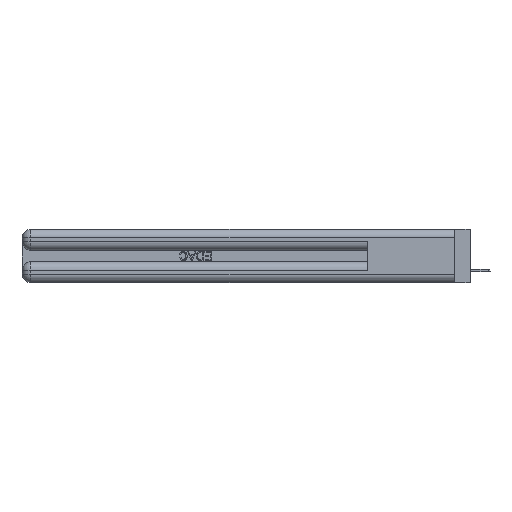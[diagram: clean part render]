
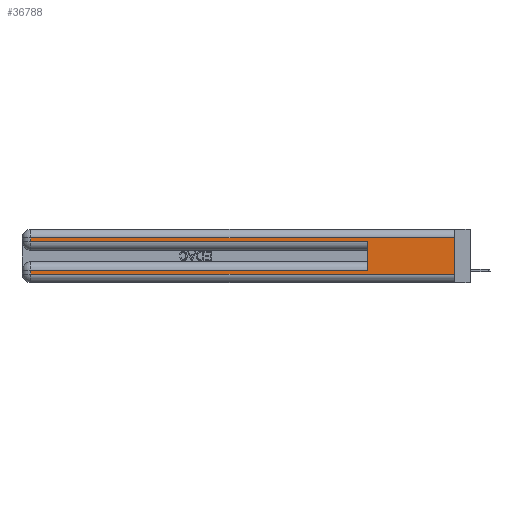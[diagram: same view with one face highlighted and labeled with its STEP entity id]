
A CAD part, left-side view. The second image highlights one B-rep face of the part: STEP entity #36788.
In plain terms, the highlighted planar face has unit normal (-1, 0, 0).
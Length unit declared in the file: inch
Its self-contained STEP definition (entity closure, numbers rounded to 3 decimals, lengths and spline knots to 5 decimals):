
#344 = CARTESIAN_POINT ( 'NONE',  ( 0., 0., 0.31 ) ) ;
#729 = CARTESIAN_POINT ( 'NONE',  ( 0., 0., 0.37 ) ) ;
#1096 = DIRECTION ( 'NONE',  ( 0., -1., 0. ) ) ;
#1603 = ORIENTED_EDGE ( 'NONE', *, *, #17889, .T. ) ;
#2224 = VERTEX_POINT ( 'NONE', #2836 ) ;
#2836 = CARTESIAN_POINT ( 'NONE',  ( 0., 0., 0.31 ) ) ;
#4087 = CARTESIAN_POINT ( 'NONE',  ( 0., 2.94, 0.06 ) ) ;
#6194 = CARTESIAN_POINT ( 'NONE',  ( 0., 2.94, 0.37 ) ) ;
#6710 = EDGE_CURVE ( 'NONE', #2224, #46949, #38378, .T. ) ;
#6787 = LINE ( 'NONE', #35916, #14885 ) ;
#9038 = EDGE_LOOP ( 'NONE', ( #23995, #1603, #45096, #53642, #51712, #34278, #30281, #24476 ) ) ;
#10480 = DIRECTION ( 'NONE',  ( 0., 1., 0. ) ) ;
#11946 = DIRECTION ( 'NONE',  ( 0., 1., 0. ) ) ;
#12211 = LINE ( 'NONE', #344, #42393 ) ;
#12593 = CARTESIAN_POINT ( 'NONE',  ( 0., 0., 0.37 ) ) ;
#14110 = EDGE_CURVE ( 'NONE', #15818, #34811, #22847, .T. ) ;
#14450 = DIRECTION ( 'NONE',  ( 0., 0., -1. ) ) ;
#14874 = EDGE_CURVE ( 'NONE', #15818, #25342, #43784, .T. ) ;
#14885 = VECTOR ( 'NONE', #52134, 39.37008 ) ;
#15342 = CARTESIAN_POINT ( 'NONE',  ( 0., 0.6, 0.085 ) ) ;
#15780 = CARTESIAN_POINT ( 'NONE',  ( 0., 0., 0.06 ) ) ;
#15818 = VERTEX_POINT ( 'NONE', #15342 ) ;
#16564 = EDGE_CURVE ( 'NONE', #39496, #46949, #45972, .T. ) ;
#17889 = EDGE_CURVE ( 'NONE', #2224, #37572, #12211, .T. ) ;
#19528 = CARTESIAN_POINT ( 'NONE',  ( 0., 0., 0.085 ) ) ;
#19926 = CARTESIAN_POINT ( 'NONE',  ( 0., 2.94, 0.285 ) ) ;
#20988 = VECTOR ( 'NONE', #1096, 39.37008 ) ;
#22847 = LINE ( 'NONE', #19528, #33501 ) ;
#23019 = VERTEX_POINT ( 'NONE', #19926 ) ;
#23995 = ORIENTED_EDGE ( 'NONE', *, *, #6710, .F. ) ;
#24476 = ORIENTED_EDGE ( 'NONE', *, *, #16564, .T. ) ;
#24909 = CARTESIAN_POINT ( 'NONE',  ( 0., 0.6, 0.285 ) ) ;
#24952 = PLANE ( 'NONE',  #43707 ) ;
#25342 = VERTEX_POINT ( 'NONE', #24909 ) ;
#26120 = CARTESIAN_POINT ( 'NONE',  ( 0., 0., 0.285 ) ) ;
#28548 = DIRECTION ( 'NONE',  ( 0., 0., -1. ) ) ;
#30281 = ORIENTED_EDGE ( 'NONE', *, *, #47200, .T. ) ;
#30934 = LINE ( 'NONE', #6194, #38969 ) ;
#33501 = VECTOR ( 'NONE', #10480, 39.37008 ) ;
#34278 = ORIENTED_EDGE ( 'NONE', *, *, #14110, .T. ) ;
#34811 = VERTEX_POINT ( 'NONE', #51135 ) ;
#35916 = CARTESIAN_POINT ( 'NONE',  ( 0., 2.94, 0.37 ) ) ;
#36788 = ADVANCED_FACE ( 'NONE', ( #50202 ), #24952, .F. ) ;
#37039 = DIRECTION ( 'NONE',  ( 1., 0., 0. ) ) ;
#37572 = VERTEX_POINT ( 'NONE', #40167 ) ;
#37828 = EDGE_CURVE ( 'NONE', #23019, #25342, #43422, .T. ) ;
#38378 = LINE ( 'NONE', #729, #45315 ) ;
#38564 = DIRECTION ( 'NONE',  ( 0., 0., 1. ) ) ;
#38969 = VECTOR ( 'NONE', #14450, 39.37008 ) ;
#39496 = VERTEX_POINT ( 'NONE', #4087 ) ;
#39715 = EDGE_CURVE ( 'NONE', #37572, #23019, #6787, .T. ) ;
#39741 = DIRECTION ( 'NONE',  ( 0., 0., -1. ) ) ;
#40167 = CARTESIAN_POINT ( 'NONE',  ( 0., 2.94, 0.31 ) ) ;
#40854 = CARTESIAN_POINT ( 'NONE',  ( 0., 0., 0.06 ) ) ;
#42393 = VECTOR ( 'NONE', #11946, 39.37008 ) ;
#43355 = VECTOR ( 'NONE', #45444, 39.37008 ) ;
#43422 = LINE ( 'NONE', #26120, #20988 ) ;
#43707 = AXIS2_PLACEMENT_3D ( 'NONE', #12593, #37039, #28548 ) ;
#43784 = LINE ( 'NONE', #52014, #44957 ) ;
#44957 = VECTOR ( 'NONE', #38564, 39.37008 ) ;
#45096 = ORIENTED_EDGE ( 'NONE', *, *, #39715, .T. ) ;
#45315 = VECTOR ( 'NONE', #39741, 39.37008 ) ;
#45444 = DIRECTION ( 'NONE',  ( 0., -1., 0. ) ) ;
#45972 = LINE ( 'NONE', #15780, #43355 ) ;
#46949 = VERTEX_POINT ( 'NONE', #40854 ) ;
#47200 = EDGE_CURVE ( 'NONE', #34811, #39496, #30934, .T. ) ;
#50202 = FACE_OUTER_BOUND ( 'NONE', #9038, .T. ) ;
#51135 = CARTESIAN_POINT ( 'NONE',  ( 0., 2.94, 0.085 ) ) ;
#51712 = ORIENTED_EDGE ( 'NONE', *, *, #14874, .F. ) ;
#52014 = CARTESIAN_POINT ( 'NONE',  ( 0., 0.6, 0.145 ) ) ;
#52134 = DIRECTION ( 'NONE',  ( 0., 0., -1. ) ) ;
#53642 = ORIENTED_EDGE ( 'NONE', *, *, #37828, .T. ) ;
